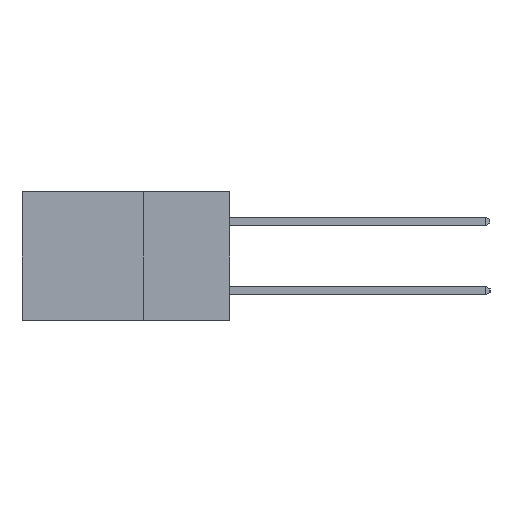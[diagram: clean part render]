
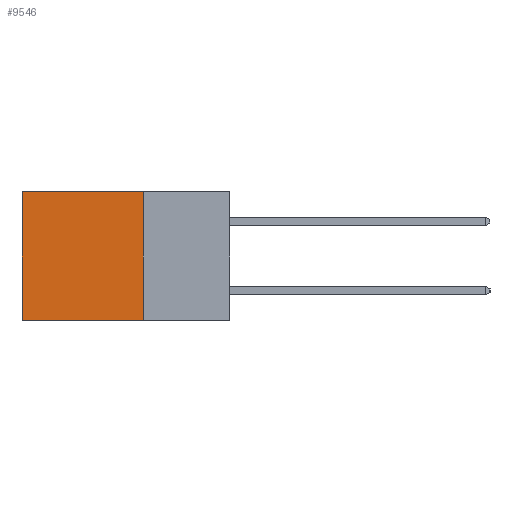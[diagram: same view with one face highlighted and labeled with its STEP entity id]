
A CAD part, left-side view. The second image highlights one B-rep face of the part: STEP entity #9546.
In plain terms, the highlighted planar face has unit normal (-1, 0, 0).
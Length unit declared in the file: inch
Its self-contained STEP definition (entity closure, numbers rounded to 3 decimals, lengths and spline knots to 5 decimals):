
#364 = LINE ( 'NONE', #7539, #6772 ) ;
#802 = VECTOR ( 'NONE', #5326, 39.37008 ) ;
#947 = VERTEX_POINT ( 'NONE', #9628 ) ;
#1288 = CARTESIAN_POINT ( 'NONE',  ( 0.2615, 0.25, -0.37 ) ) ;
#1700 = EDGE_LOOP ( 'NONE', ( #4248, #10387, #6708, #3512 ) ) ;
#2289 = EDGE_CURVE ( 'NONE', #6675, #6512, #364, .T. ) ;
#2562 = VECTOR ( 'NONE', #4115, 39.37008 ) ;
#3433 = FACE_OUTER_BOUND ( 'NONE', #1700, .T. ) ;
#3512 = ORIENTED_EDGE ( 'NONE', *, *, #2289, .T. ) ;
#3739 = EDGE_CURVE ( 'NONE', #947, #9993, #10595, .T. ) ;
#3751 = DIRECTION ( 'NONE',  ( 0., 1., 0. ) ) ;
#3851 = LINE ( 'NONE', #5455, #802 ) ;
#3936 = CARTESIAN_POINT ( 'NONE',  ( 0.2615, 0.25, -0.37 ) ) ;
#3996 = VECTOR ( 'NONE', #3751, 39.37008 ) ;
#4115 = DIRECTION ( 'NONE',  ( 0., 0., -1. ) ) ;
#4248 = ORIENTED_EDGE ( 'NONE', *, *, #9171, .T. ) ;
#4294 = DIRECTION ( 'NONE',  ( 0., 1., 0. ) ) ;
#4753 = EDGE_CURVE ( 'NONE', #6675, #947, #9202, .T. ) ;
#5326 = DIRECTION ( 'NONE',  ( 0., 0., -1. ) ) ;
#5455 = CARTESIAN_POINT ( 'NONE',  ( 0.2615, 0.6, -0.37 ) ) ;
#6512 = VERTEX_POINT ( 'NONE', #13772 ) ;
#6675 = VERTEX_POINT ( 'NONE', #12229 ) ;
#6708 = ORIENTED_EDGE ( 'NONE', *, *, #4753, .F. ) ;
#6772 = VECTOR ( 'NONE', #4294, 39.37008 ) ;
#7539 = CARTESIAN_POINT ( 'NONE',  ( 0.2615, 0.25, 0. ) ) ;
#9171 = EDGE_CURVE ( 'NONE', #6512, #9993, #3851, .T. ) ;
#9202 = LINE ( 'NONE', #1288, #2562 ) ;
#9546 = ADVANCED_FACE ( 'NONE', ( #3433 ), #14838, .F. ) ;
#9628 = CARTESIAN_POINT ( 'NONE',  ( 0.2615, 0.25, -0.37 ) ) ;
#9993 = VERTEX_POINT ( 'NONE', #11522 ) ;
#10387 = ORIENTED_EDGE ( 'NONE', *, *, #3739, .F. ) ;
#10595 = LINE ( 'NONE', #3936, #3996 ) ;
#11522 = CARTESIAN_POINT ( 'NONE',  ( 0.2615, 0.6, -0.37 ) ) ;
#12152 = AXIS2_PLACEMENT_3D ( 'NONE', #14707, #14697, #14681 ) ;
#12229 = CARTESIAN_POINT ( 'NONE',  ( 0.2615, 0.25, 0. ) ) ;
#13772 = CARTESIAN_POINT ( 'NONE',  ( 0.2615, 0.6, 0. ) ) ;
#14681 = DIRECTION ( 'NONE',  ( 0., 0., -1. ) ) ;
#14697 = DIRECTION ( 'NONE',  ( 1., 0., 0. ) ) ;
#14707 = CARTESIAN_POINT ( 'NONE',  ( 0.2615, 0.25, -0.37 ) ) ;
#14838 = PLANE ( 'NONE',  #12152 ) ;
